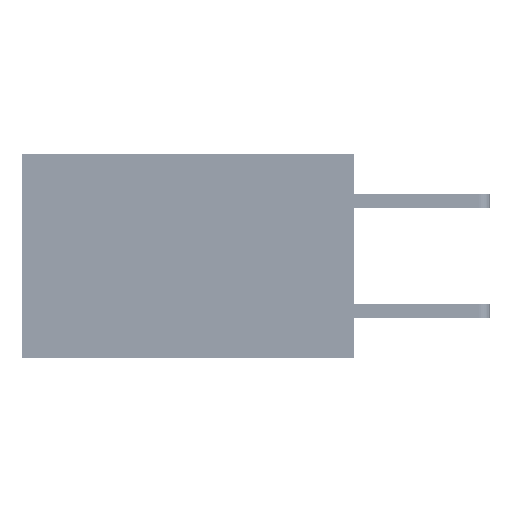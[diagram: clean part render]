
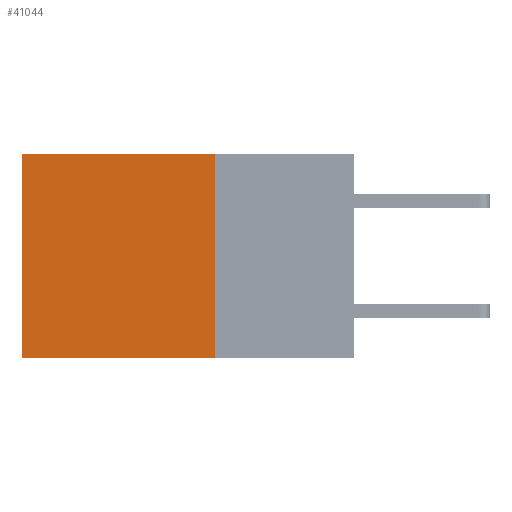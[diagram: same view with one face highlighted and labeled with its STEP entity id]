
A CAD part, left-side view. The second image highlights one B-rep face of the part: STEP entity #41044.
In plain terms, the highlighted planar face has unit normal (-1, 0, 0).
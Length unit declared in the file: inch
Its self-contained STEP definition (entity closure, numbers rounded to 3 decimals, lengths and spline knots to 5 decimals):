
#4831 = CARTESIAN_POINT ( 'NONE',  ( 0.2875, 0.25, 0. ) ) ;
#5375 = DIRECTION ( 'NONE',  ( 0., 0., -1. ) ) ;
#5571 = DIRECTION ( 'NONE',  ( 0., 1., 0. ) ) ;
#5952 = DIRECTION ( 'NONE',  ( 0., 1., 0. ) ) ;
#7496 = DIRECTION ( 'NONE',  ( 0., 0., -1. ) ) ;
#7940 = EDGE_CURVE ( 'NONE', #29030, #13662, #26176, .T. ) ;
#11768 = VERTEX_POINT ( 'NONE', #43172 ) ;
#12285 = CARTESIAN_POINT ( 'NONE',  ( 0.2875, 0.6, -0.37 ) ) ;
#13662 = VERTEX_POINT ( 'NONE', #12285 ) ;
#16224 = ORIENTED_EDGE ( 'NONE', *, *, #39767, .T. ) ;
#16555 = LINE ( 'NONE', #4831, #39006 ) ;
#17561 = LINE ( 'NONE', #25257, #46292 ) ;
#17892 = EDGE_CURVE ( 'NONE', #11768, #29030, #16555, .T. ) ;
#19763 = DIRECTION ( 'NONE',  ( 1., 0., 0. ) ) ;
#24435 = CARTESIAN_POINT ( 'NONE',  ( 0.2875, 0.25, -0.37 ) ) ;
#25257 = CARTESIAN_POINT ( 'NONE',  ( 0.2875, 0.25, 0. ) ) ;
#26176 = LINE ( 'NONE', #42337, #34768 ) ;
#26599 = DIRECTION ( 'NONE',  ( 0., 0., -1. ) ) ;
#29030 = VERTEX_POINT ( 'NONE', #24435 ) ;
#30061 = LINE ( 'NONE', #30839, #35895 ) ;
#30839 = CARTESIAN_POINT ( 'NONE',  ( 0.2875, 0.6, 0. ) ) ;
#34768 = VECTOR ( 'NONE', #5952, 39.37008 ) ;
#35895 = VECTOR ( 'NONE', #26599, 39.37008 ) ;
#39006 = VECTOR ( 'NONE', #5375, 39.37008 ) ;
#39014 = CARTESIAN_POINT ( 'NONE',  ( 0.2875, 0.6, 0. ) ) ;
#39767 = EDGE_CURVE ( 'NONE', #41728, #13662, #30061, .T. ) ;
#39903 = ORIENTED_EDGE ( 'NONE', *, *, #7940, .F. ) ;
#39913 = CARTESIAN_POINT ( 'NONE',  ( 0.2875, 0.25, 0. ) ) ;
#40951 = FACE_OUTER_BOUND ( 'NONE', #47586, .T. ) ;
#41044 = ADVANCED_FACE ( 'NONE', ( #40951 ), #48116, .F. ) ;
#41728 = VERTEX_POINT ( 'NONE', #39014 ) ;
#42337 = CARTESIAN_POINT ( 'NONE',  ( 0.2875, 0.25, -0.37 ) ) ;
#42955 = EDGE_CURVE ( 'NONE', #11768, #41728, #17561, .T. ) ;
#43172 = CARTESIAN_POINT ( 'NONE',  ( 0.2875, 0.25, 0. ) ) ;
#45035 = ORIENTED_EDGE ( 'NONE', *, *, #42955, .T. ) ;
#46292 = VECTOR ( 'NONE', #5571, 39.37008 ) ;
#47586 = EDGE_LOOP ( 'NONE', ( #16224, #39903, #48096, #45035 ) ) ;
#48096 = ORIENTED_EDGE ( 'NONE', *, *, #17892, .F. ) ;
#48116 = PLANE ( 'NONE',  #50441 ) ;
#50441 = AXIS2_PLACEMENT_3D ( 'NONE', #39913, #19763, #7496 ) ;
